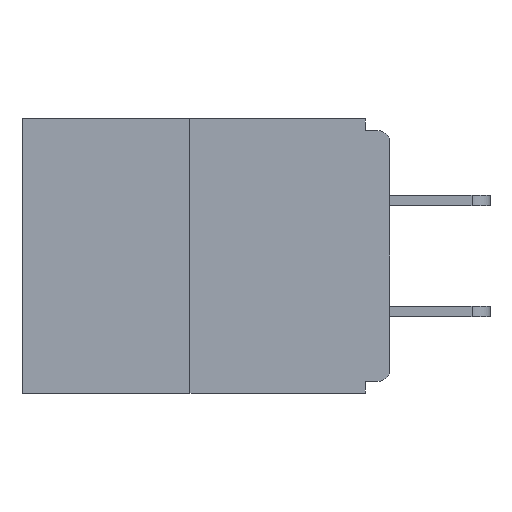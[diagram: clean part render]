
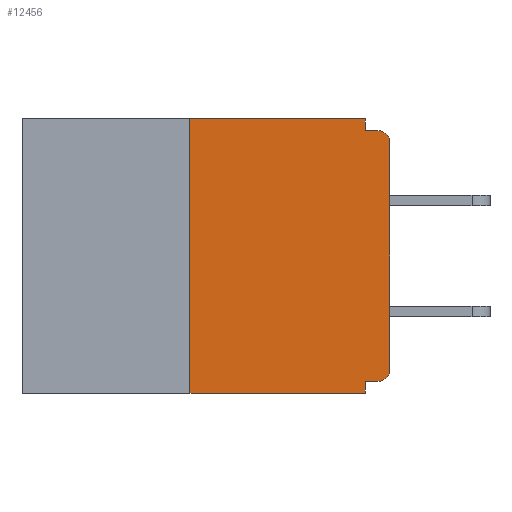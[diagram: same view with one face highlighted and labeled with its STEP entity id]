
A CAD part, left-side view. The second image highlights one B-rep face of the part: STEP entity #12456.
In plain terms, the highlighted planar face has unit normal (-1, 0, 0).
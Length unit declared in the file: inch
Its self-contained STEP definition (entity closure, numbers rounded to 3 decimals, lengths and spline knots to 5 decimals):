
#4 = VECTOR ( 'NONE', #4381, 39.37008 ) ;
#209 = EDGE_CURVE ( 'NONE', #7728, #5365, #12523, .T. ) ;
#282 = CARTESIAN_POINT ( 'NONE',  ( 0., 0.031, -0.328 ) ) ;
#788 = PLANE ( 'NONE',  #4376 ) ;
#819 = VECTOR ( 'NONE', #1290, 39.37008 ) ;
#1290 = DIRECTION ( 'NONE',  ( 0., -1., 0. ) ) ;
#1524 = DIRECTION ( 'NONE',  ( 0., 0., -1. ) ) ;
#1702 = AXIS2_PLACEMENT_3D ( 'NONE', #19189, #2536, #4497 ) ;
#1715 = CARTESIAN_POINT ( 'NONE',  ( 0., 0., -0.03 ) ) ;
#2023 = EDGE_CURVE ( 'NONE', #21312, #14688, #8521, .T. ) ;
#2030 = CARTESIAN_POINT ( 'NONE',  ( 0., 0., -0.328 ) ) ;
#2474 = LINE ( 'NONE', #7519, #20302 ) ;
#2536 = DIRECTION ( 'NONE',  ( -1., 0., 0. ) ) ;
#2708 = VECTOR ( 'NONE', #20430, 39.37008 ) ;
#3035 = DIRECTION ( 'NONE',  ( -1., 0., 0. ) ) ;
#3282 = CARTESIAN_POINT ( 'NONE',  ( 0., 0.015, -0.328 ) ) ;
#3572 = EDGE_LOOP ( 'NONE', ( #13346, #21326, #10119, #13073, #12242, #14055, #17300, #19309, #17128, #13513 ) ) ;
#3792 = LINE ( 'NONE', #5183, #19535 ) ;
#4125 = AXIS2_PLACEMENT_3D ( 'NONE', #6346, #3035, #1524 ) ;
#4376 = AXIS2_PLACEMENT_3D ( 'NONE', #16011, #15946, #17769 ) ;
#4381 = DIRECTION ( 'NONE',  ( 0., 0., 1. ) ) ;
#4497 = DIRECTION ( 'NONE',  ( 0., 0., -1. ) ) ;
#4648 = VECTOR ( 'NONE', #20264, 39.37008 ) ;
#5183 = CARTESIAN_POINT ( 'NONE',  ( 0., 0.031, -0.343 ) ) ;
#5365 = VERTEX_POINT ( 'NONE', #11809 ) ;
#5875 = VERTEX_POINT ( 'NONE', #16885 ) ;
#6286 = CARTESIAN_POINT ( 'NONE',  ( 0., 0.031, -0.343 ) ) ;
#6346 = CARTESIAN_POINT ( 'NONE',  ( 0., 0.015, -0.03 ) ) ;
#6586 = CIRCLE ( 'NONE', #1702, 0.015 ) ;
#7041 = CARTESIAN_POINT ( 'NONE',  ( 0., 0.46, 0. ) ) ;
#7265 = VERTEX_POINT ( 'NONE', #10036 ) ;
#7519 = CARTESIAN_POINT ( 'NONE',  ( 0., 0.25, 0. ) ) ;
#7728 = VERTEX_POINT ( 'NONE', #8397 ) ;
#8217 = LINE ( 'NONE', #7041, #20845 ) ;
#8397 = CARTESIAN_POINT ( 'NONE',  ( 0., 0.031, 0. ) ) ;
#8521 = LINE ( 'NONE', #2030, #4648 ) ;
#10036 = CARTESIAN_POINT ( 'NONE',  ( 0., 0., -0.313 ) ) ;
#10119 = ORIENTED_EDGE ( 'NONE', *, *, #15954, .T. ) ;
#10328 = VERTEX_POINT ( 'NONE', #19868 ) ;
#10342 = CARTESIAN_POINT ( 'NONE',  ( 0., 0., -0.015 ) ) ;
#10840 = DIRECTION ( 'NONE',  ( 0., 0., 1. ) ) ;
#11809 = CARTESIAN_POINT ( 'NONE',  ( 0., 0.031, -0.015 ) ) ;
#12242 = ORIENTED_EDGE ( 'NONE', *, *, #2023, .F. ) ;
#12314 = VECTOR ( 'NONE', #20218, 39.37008 ) ;
#12456 = ADVANCED_FACE ( 'NONE', ( #14000 ), #788, .F. ) ;
#12459 = CARTESIAN_POINT ( 'NONE',  ( 0., 0., 0. ) ) ;
#12523 = LINE ( 'NONE', #17037, #2708 ) ;
#13073 = ORIENTED_EDGE ( 'NONE', *, *, #20080, .F. ) ;
#13346 = ORIENTED_EDGE ( 'NONE', *, *, #17776, .F. ) ;
#13513 = ORIENTED_EDGE ( 'NONE', *, *, #209, .F. ) ;
#13846 = DIRECTION ( 'NONE',  ( 0., -1., 0. ) ) ;
#13919 = EDGE_CURVE ( 'NONE', #16742, #5875, #14515, .T. ) ;
#14000 = FACE_OUTER_BOUND ( 'NONE', #3572, .T. ) ;
#14055 = ORIENTED_EDGE ( 'NONE', *, *, #18726, .T. ) ;
#14515 = CIRCLE ( 'NONE', #4125, 0.015 ) ;
#14688 = VERTEX_POINT ( 'NONE', #282 ) ;
#14855 = CARTESIAN_POINT ( 'NONE',  ( 0., 0.25, 0. ) ) ;
#15125 = VERTEX_POINT ( 'NONE', #14855 ) ;
#15946 = DIRECTION ( 'NONE',  ( 1., 0., 0. ) ) ;
#15954 = EDGE_CURVE ( 'NONE', #10328, #18976, #18077, .T. ) ;
#16011 = CARTESIAN_POINT ( 'NONE',  ( 0., 0.46, 0. ) ) ;
#16172 = CARTESIAN_POINT ( 'NONE',  ( 0., 0.46, -0.343 ) ) ;
#16415 = EDGE_CURVE ( 'NONE', #7265, #16742, #17009, .T. ) ;
#16584 = DIRECTION ( 'NONE',  ( 0., 0., -1. ) ) ;
#16742 = VERTEX_POINT ( 'NONE', #1715 ) ;
#16885 = CARTESIAN_POINT ( 'NONE',  ( 0., 0.015, -0.015 ) ) ;
#17009 = LINE ( 'NONE', #12459, #4 ) ;
#17037 = CARTESIAN_POINT ( 'NONE',  ( 0., 0.031, 0. ) ) ;
#17128 = ORIENTED_EDGE ( 'NONE', *, *, #18029, .F. ) ;
#17300 = ORIENTED_EDGE ( 'NONE', *, *, #16415, .T. ) ;
#17769 = DIRECTION ( 'NONE',  ( 0., 0., -1. ) ) ;
#17776 = EDGE_CURVE ( 'NONE', #15125, #7728, #8217, .T. ) ;
#18029 = EDGE_CURVE ( 'NONE', #5365, #5875, #19534, .T. ) ;
#18077 = LINE ( 'NONE', #16172, #819 ) ;
#18282 = EDGE_CURVE ( 'NONE', #10328, #15125, #2474, .T. ) ;
#18726 = EDGE_CURVE ( 'NONE', #21312, #7265, #6586, .T. ) ;
#18976 = VERTEX_POINT ( 'NONE', #6286 ) ;
#19189 = CARTESIAN_POINT ( 'NONE',  ( 0., 0.015, -0.313 ) ) ;
#19309 = ORIENTED_EDGE ( 'NONE', *, *, #13919, .T. ) ;
#19534 = LINE ( 'NONE', #10342, #12314 ) ;
#19535 = VECTOR ( 'NONE', #16584, 39.37008 ) ;
#19868 = CARTESIAN_POINT ( 'NONE',  ( 0., 0.25, -0.343 ) ) ;
#20080 = EDGE_CURVE ( 'NONE', #14688, #18976, #3792, .T. ) ;
#20218 = DIRECTION ( 'NONE',  ( 0., -1., 0. ) ) ;
#20264 = DIRECTION ( 'NONE',  ( 0., 1., 0. ) ) ;
#20302 = VECTOR ( 'NONE', #10840, 39.37008 ) ;
#20430 = DIRECTION ( 'NONE',  ( 0., 0., -1. ) ) ;
#20845 = VECTOR ( 'NONE', #13846, 39.37008 ) ;
#21312 = VERTEX_POINT ( 'NONE', #3282 ) ;
#21326 = ORIENTED_EDGE ( 'NONE', *, *, #18282, .F. ) ;
